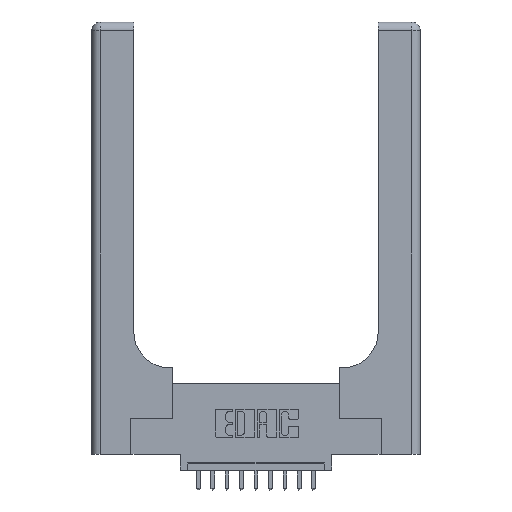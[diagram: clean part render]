
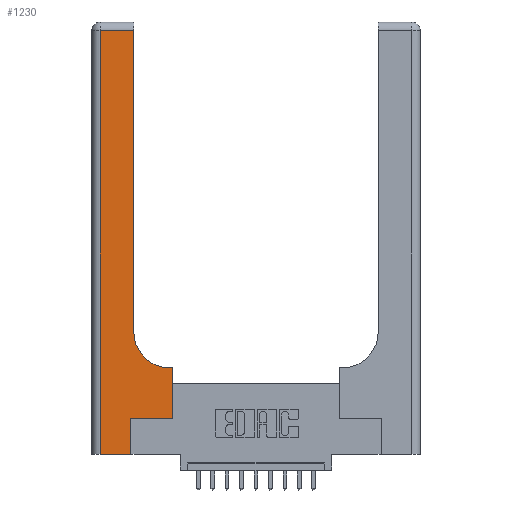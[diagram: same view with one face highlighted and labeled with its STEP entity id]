
A CAD part, top view. The second image highlights one B-rep face of the part: STEP entity #1230.
In plain terms, the highlighted planar face has unit normal (0, 0, 1).
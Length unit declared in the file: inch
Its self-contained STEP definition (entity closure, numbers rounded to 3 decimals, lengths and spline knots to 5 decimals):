
#289 = EDGE_CURVE ( 'NONE', #4131, #11479, #10945, .T. ) ;
#427 = CARTESIAN_POINT ( 'NONE',  ( 0.2915, 0.6, 0.37 ) ) ;
#462 = EDGE_CURVE ( 'NONE', #15136, #8582, #772, .T. ) ;
#656 = VECTOR ( 'NONE', #9470, 39.37008 ) ;
#772 = LINE ( 'NONE', #3843, #16136 ) ;
#808 = VERTEX_POINT ( 'NONE', #7302 ) ;
#879 = DIRECTION ( 'NONE',  ( 0., 0., -1. ) ) ;
#1118 = CARTESIAN_POINT ( 'NONE',  ( 0.5585, 0.25, 0.37 ) ) ;
#1151 = CARTESIAN_POINT ( 'NONE',  ( 0.5585, 0.6, 0.37 ) ) ;
#1230 = ADVANCED_FACE ( 'NONE', ( #11736 ), #12228, .F. ) ;
#1238 = EDGE_CURVE ( 'NONE', #11298, #4131, #12331, .T. ) ;
#1328 = DIRECTION ( 'NONE',  ( -1., 0., 0. ) ) ;
#1615 = CARTESIAN_POINT ( 'NONE',  ( 0.2915, 3., 0.37 ) ) ;
#2030 = DIRECTION ( 'NONE',  ( 0., 1., 0. ) ) ;
#2180 = DIRECTION ( 'NONE',  ( -1., 0., 0. ) ) ;
#2191 = ORIENTED_EDGE ( 'NONE', *, *, #1238, .T. ) ;
#2437 = CIRCLE ( 'NONE', #7975, 0.25 ) ;
#2584 = CARTESIAN_POINT ( 'NONE',  ( 0.269, 0., 0.37 ) ) ;
#2970 = LINE ( 'NONE', #1118, #13356 ) ;
#3735 = DIRECTION ( 'NONE',  ( 0., 1., 0. ) ) ;
#3843 = CARTESIAN_POINT ( 'NONE',  ( 0., 2.94, 0.37 ) ) ;
#3910 = CARTESIAN_POINT ( 'NONE',  ( 0.269, 0.25, 0.37 ) ) ;
#4036 = LINE ( 'NONE', #1615, #656 ) ;
#4111 = ORIENTED_EDGE ( 'NONE', *, *, #6454, .T. ) ;
#4131 = VERTEX_POINT ( 'NONE', #2584 ) ;
#4326 = CARTESIAN_POINT ( 'NONE',  ( 0.269, 0.25, 0.37 ) ) ;
#6014 = VECTOR ( 'NONE', #10582, 39.37008 ) ;
#6250 = CARTESIAN_POINT ( 'NONE',  ( 0.06, 0., 0.37 ) ) ;
#6310 = VECTOR ( 'NONE', #2030, 39.37008 ) ;
#6404 = LINE ( 'NONE', #427, #6014 ) ;
#6454 = EDGE_CURVE ( 'NONE', #11091, #12682, #2970, .T. ) ;
#6840 = EDGE_LOOP ( 'NONE', ( #16245, #13526, #8166, #2191, #9429, #14446, #4111, #16273, #15785 ) ) ;
#7302 = CARTESIAN_POINT ( 'NONE',  ( 0.5415, 0.6, 0.37 ) ) ;
#7400 = CARTESIAN_POINT ( 'NONE',  ( 0.5585, 0.25, 0.37 ) ) ;
#7975 = AXIS2_PLACEMENT_3D ( 'NONE', #11029, #879, #12333 ) ;
#8159 = EDGE_CURVE ( 'NONE', #11479, #11091, #14510, .T. ) ;
#8166 = ORIENTED_EDGE ( 'NONE', *, *, #9901, .T. ) ;
#8582 = VERTEX_POINT ( 'NONE', #11863 ) ;
#9429 = ORIENTED_EDGE ( 'NONE', *, *, #289, .T. ) ;
#9445 = EDGE_CURVE ( 'NONE', #9719, #15136, #4036, .T. ) ;
#9470 = DIRECTION ( 'NONE',  ( 0., 1., 0. ) ) ;
#9482 = EDGE_CURVE ( 'NONE', #12682, #808, #6404, .T. ) ;
#9719 = VERTEX_POINT ( 'NONE', #9980 ) ;
#9901 = EDGE_CURVE ( 'NONE', #8582, #11298, #12231, .T. ) ;
#9955 = AXIS2_PLACEMENT_3D ( 'NONE', #15796, #12394, #2180 ) ;
#9980 = CARTESIAN_POINT ( 'NONE',  ( 0.2915, 0.85, 0.37 ) ) ;
#10118 = VECTOR ( 'NONE', #11036, 39.37008 ) ;
#10129 = DIRECTION ( 'NONE',  ( 0., -1., 0. ) ) ;
#10442 = CARTESIAN_POINT ( 'NONE',  ( 0.2915, 2.94, 0.37 ) ) ;
#10488 = VECTOR ( 'NONE', #15416, 39.37008 ) ;
#10582 = DIRECTION ( 'NONE',  ( -1., 0., 0. ) ) ;
#10945 = LINE ( 'NONE', #15983, #6310 ) ;
#11029 = CARTESIAN_POINT ( 'NONE',  ( 0.5415, 0.85, 0.37 ) ) ;
#11036 = DIRECTION ( 'NONE',  ( 1., 0., 0. ) ) ;
#11091 = VERTEX_POINT ( 'NONE', #7400 ) ;
#11298 = VERTEX_POINT ( 'NONE', #6250 ) ;
#11479 = VERTEX_POINT ( 'NONE', #4326 ) ;
#11736 = FACE_OUTER_BOUND ( 'NONE', #6840, .T. ) ;
#11863 = CARTESIAN_POINT ( 'NONE',  ( 0.06, 2.94, 0.37 ) ) ;
#12228 = PLANE ( 'NONE',  #9955 ) ;
#12231 = LINE ( 'NONE', #13944, #15811 ) ;
#12331 = LINE ( 'NONE', #16222, #10118 ) ;
#12333 = DIRECTION ( 'NONE',  ( 1., 0., 0. ) ) ;
#12394 = DIRECTION ( 'NONE',  ( 0., 0., -1. ) ) ;
#12682 = VERTEX_POINT ( 'NONE', #1151 ) ;
#13356 = VECTOR ( 'NONE', #3735, 39.37008 ) ;
#13526 = ORIENTED_EDGE ( 'NONE', *, *, #462, .T. ) ;
#13944 = CARTESIAN_POINT ( 'NONE',  ( 0.06, 3., 0.37 ) ) ;
#14446 = ORIENTED_EDGE ( 'NONE', *, *, #8159, .T. ) ;
#14510 = LINE ( 'NONE', #3910, #10488 ) ;
#15136 = VERTEX_POINT ( 'NONE', #10442 ) ;
#15377 = EDGE_CURVE ( 'NONE', #808, #9719, #2437, .T. ) ;
#15416 = DIRECTION ( 'NONE',  ( 1., 0., 0. ) ) ;
#15785 = ORIENTED_EDGE ( 'NONE', *, *, #15377, .T. ) ;
#15796 = CARTESIAN_POINT ( 'NONE',  ( 0., 3., 0.37 ) ) ;
#15811 = VECTOR ( 'NONE', #10129, 39.37008 ) ;
#15983 = CARTESIAN_POINT ( 'NONE',  ( 0.269, 0., 0.37 ) ) ;
#16136 = VECTOR ( 'NONE', #1328, 39.37008 ) ;
#16222 = CARTESIAN_POINT ( 'NONE',  ( 0., 0., 0.37 ) ) ;
#16245 = ORIENTED_EDGE ( 'NONE', *, *, #9445, .T. ) ;
#16273 = ORIENTED_EDGE ( 'NONE', *, *, #9482, .T. ) ;
